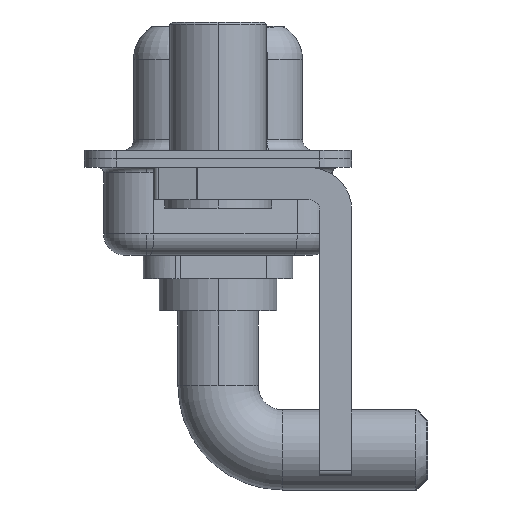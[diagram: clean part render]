
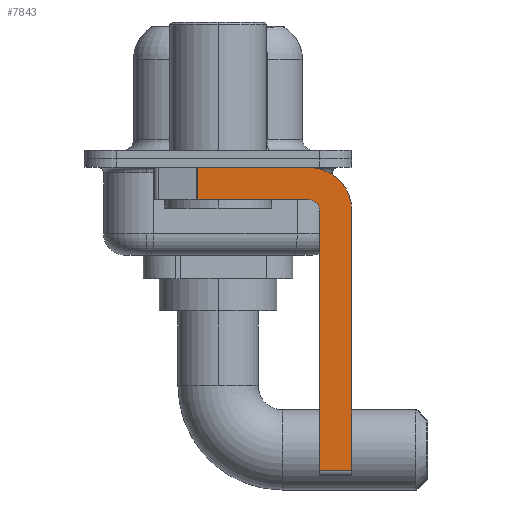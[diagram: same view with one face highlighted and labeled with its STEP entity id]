
A CAD part, left-side view. The second image highlights one B-rep face of the part: STEP entity #7843.
In plain terms, the highlighted planar face has unit normal (-1, 0, 0).
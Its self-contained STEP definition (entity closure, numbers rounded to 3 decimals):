
#145 = ORIENTED_EDGE ( 'NONE', *, *, #8326, .F. ) ;
#422 = VERTEX_POINT ( 'NONE', #13899 ) ;
#767 = VERTEX_POINT ( 'NONE', #14962 ) ;
#952 = DIRECTION ( 'NONE',  ( 0., 0., -1. ) ) ;
#984 = CARTESIAN_POINT ( 'NONE',  ( -2.9, -4.75, -14.8 ) ) ;
#990 = DIRECTION ( 'NONE',  ( 0., 0., -1. ) ) ;
#1067 = VECTOR ( 'NONE', #15304, 1000. ) ;
#1113 = CARTESIAN_POINT ( 'NONE',  ( -2.9, -4.25, -14.55 ) ) ;
#1146 = DIRECTION ( 'NONE',  ( 0., 0., 1. ) ) ;
#1289 = CARTESIAN_POINT ( 'NONE',  ( -2.9, -4.25, -1.9 ) ) ;
#1292 = PLANE ( 'NONE',  #14722 ) ;
#1347 = CARTESIAN_POINT ( 'NONE',  ( -2.9, -4.25, -2.4 ) ) ;
#1661 = EDGE_CURVE ( 'NONE', #9250, #767, #8764, .T. ) ;
#2838 = VERTEX_POINT ( 'NONE', #8387 ) ;
#3061 = VECTOR ( 'NONE', #1146, 1000. ) ;
#3429 = EDGE_CURVE ( 'NONE', #2838, #10481, #8053, .T. ) ;
#3504 = CARTESIAN_POINT ( 'NONE',  ( -2.9, 0.978, -1.9 ) ) ;
#3849 = CARTESIAN_POINT ( 'NONE',  ( -2.9, -4.25, -2.4 ) ) ;
#3930 = DIRECTION ( 'NONE',  ( 0., 0., -1. ) ) ;
#4218 = CARTESIAN_POINT ( 'NONE',  ( -2.9, -4.25, -2.4 ) ) ;
#4371 = EDGE_CURVE ( 'NONE', #9250, #15483, #7497, .T. ) ;
#4383 = ORIENTED_EDGE ( 'NONE', *, *, #1661, .T. ) ;
#5322 = DIRECTION ( 'NONE',  ( 0., 0., 1. ) ) ;
#5509 = CARTESIAN_POINT ( 'NONE',  ( -2.9, -4.75, -2.4 ) ) ;
#6193 = ORIENTED_EDGE ( 'NONE', *, *, #3429, .F. ) ;
#6939 = VERTEX_POINT ( 'NONE', #1289 ) ;
#6989 = CARTESIAN_POINT ( 'NONE',  ( -2.9, -6.25, -2.4 ) ) ;
#7084 = VECTOR ( 'NONE', #12747, 1000. ) ;
#7497 = LINE ( 'NONE', #984, #3061 ) ;
#7698 = DIRECTION ( 'NONE',  ( -1., 0., 0. ) ) ;
#7843 = ADVANCED_FACE ( 'NONE', ( #12768 ), #1292, .F. ) ;
#8019 = VECTOR ( 'NONE', #16207, 1000. ) ;
#8053 = CIRCLE ( 'NONE', #12022, 2. ) ;
#8124 = EDGE_CURVE ( 'NONE', #422, #16130, #14822, .T. ) ;
#8325 = EDGE_CURVE ( 'NONE', #15483, #6939, #13937, .T. ) ;
#8326 = EDGE_CURVE ( 'NONE', #422, #2838, #12501, .T. ) ;
#8387 = CARTESIAN_POINT ( 'NONE',  ( -2.9, -4.25, -0.4 ) ) ;
#8764 = LINE ( 'NONE', #1113, #8019 ) ;
#9194 = CARTESIAN_POINT ( 'NONE',  ( -2.9, -4.75, -14.55 ) ) ;
#9250 = VERTEX_POINT ( 'NONE', #9194 ) ;
#9682 = EDGE_CURVE ( 'NONE', #6939, #16130, #10250, .T. ) ;
#10250 = LINE ( 'NONE', #10330, #1067 ) ;
#10330 = CARTESIAN_POINT ( 'NONE',  ( -2.9, -4.25, -1.9 ) ) ;
#10481 = VERTEX_POINT ( 'NONE', #6989 ) ;
#10949 = LINE ( 'NONE', #12129, #11415 ) ;
#11268 = CARTESIAN_POINT ( 'NONE',  ( -2.9, 0.978, -1.9 ) ) ;
#11282 = EDGE_LOOP ( 'NONE', ( #145, #13173, #11827, #16205, #13526, #4383, #16031, #6193 ) ) ;
#11415 = VECTOR ( 'NONE', #990, 1000. ) ;
#11607 = DIRECTION ( 'NONE',  ( 1., 0., 0. ) ) ;
#11811 = DIRECTION ( 'NONE',  ( 1., 0., 0. ) ) ;
#11827 = ORIENTED_EDGE ( 'NONE', *, *, #9682, .F. ) ;
#12022 = AXIS2_PLACEMENT_3D ( 'NONE', #4218, #11811, #14204 ) ;
#12129 = CARTESIAN_POINT ( 'NONE',  ( -2.9, -6.25, -2.4 ) ) ;
#12501 = LINE ( 'NONE', #14060, #7084 ) ;
#12747 = DIRECTION ( 'NONE',  ( 0., -1., 0. ) ) ;
#12768 = FACE_OUTER_BOUND ( 'NONE', #11282, .T. ) ;
#13173 = ORIENTED_EDGE ( 'NONE', *, *, #8124, .T. ) ;
#13526 = ORIENTED_EDGE ( 'NONE', *, *, #4371, .F. ) ;
#13899 = CARTESIAN_POINT ( 'NONE',  ( -2.9, 0.978, -0.4 ) ) ;
#13937 = CIRCLE ( 'NONE', #15258, 0.5 ) ;
#14060 = CARTESIAN_POINT ( 'NONE',  ( -2.9, 3., -0.4 ) ) ;
#14204 = DIRECTION ( 'NONE',  ( 0., 0., -1. ) ) ;
#14722 = AXIS2_PLACEMENT_3D ( 'NONE', #3849, #11607, #3930 ) ;
#14822 = LINE ( 'NONE', #3504, #16296 ) ;
#14962 = CARTESIAN_POINT ( 'NONE',  ( -2.9, -6.25, -14.55 ) ) ;
#15207 = EDGE_CURVE ( 'NONE', #10481, #767, #10949, .T. ) ;
#15258 = AXIS2_PLACEMENT_3D ( 'NONE', #1347, #7698, #5322 ) ;
#15304 = DIRECTION ( 'NONE',  ( 0., 1., 0. ) ) ;
#15483 = VERTEX_POINT ( 'NONE', #5509 ) ;
#16031 = ORIENTED_EDGE ( 'NONE', *, *, #15207, .F. ) ;
#16130 = VERTEX_POINT ( 'NONE', #11268 ) ;
#16205 = ORIENTED_EDGE ( 'NONE', *, *, #8325, .F. ) ;
#16207 = DIRECTION ( 'NONE',  ( 0., -1., 0. ) ) ;
#16296 = VECTOR ( 'NONE', #952, 1000. ) ;
